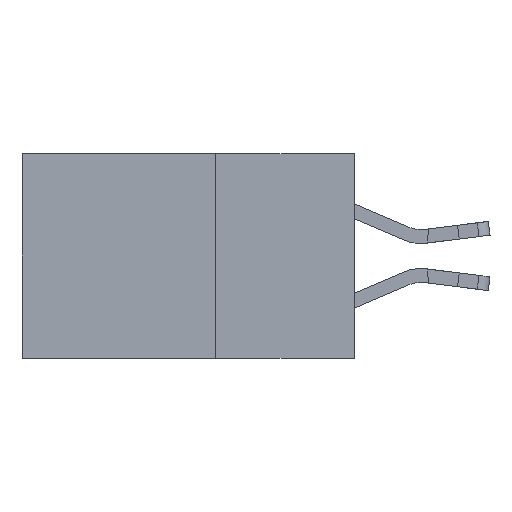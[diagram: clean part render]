
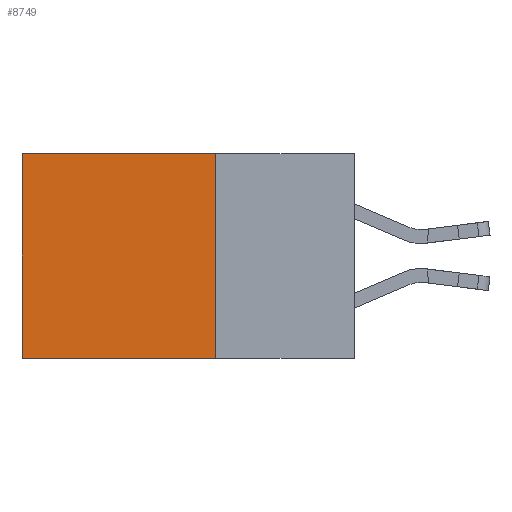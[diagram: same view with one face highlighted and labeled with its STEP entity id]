
A CAD part, left-side view. The second image highlights one B-rep face of the part: STEP entity #8749.
In plain terms, the highlighted planar face has unit normal (-1, 0, 0).
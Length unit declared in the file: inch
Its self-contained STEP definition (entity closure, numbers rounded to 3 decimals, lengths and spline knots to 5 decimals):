
#829 = EDGE_CURVE ( 'NONE', #6192, #14284, #8144, .T. ) ;
#2769 = CARTESIAN_POINT ( 'NONE',  ( 0.298, 0.6, -0.37 ) ) ;
#3401 = CARTESIAN_POINT ( 'NONE',  ( 0.298, 0.25, 0. ) ) ;
#4097 = LINE ( 'NONE', #3401, #11950 ) ;
#4464 = CARTESIAN_POINT ( 'NONE',  ( 0.298, 0.6, 0. ) ) ;
#4485 = LINE ( 'NONE', #6774, #6534 ) ;
#4515 = EDGE_CURVE ( 'NONE', #8010, #6192, #4485, .T. ) ;
#5329 = DIRECTION ( 'NONE',  ( 0., 1., 0. ) ) ;
#5430 = CARTESIAN_POINT ( 'NONE',  ( 0.298, 0.25, 0. ) ) ;
#6192 = VERTEX_POINT ( 'NONE', #6195 ) ;
#6195 = CARTESIAN_POINT ( 'NONE',  ( 0.298, 0.25, -0.37 ) ) ;
#6402 = CARTESIAN_POINT ( 'NONE',  ( 0.298, 0.6, 0. ) ) ;
#6466 = EDGE_CURVE ( 'NONE', #9532, #14284, #6539, .T. ) ;
#6534 = VECTOR ( 'NONE', #7986, 39.37008 ) ;
#6539 = LINE ( 'NONE', #4464, #15147 ) ;
#6612 = DIRECTION ( 'NONE',  ( 1., 0., 0. ) ) ;
#6774 = CARTESIAN_POINT ( 'NONE',  ( 0.298, 0.25, 0. ) ) ;
#6799 = EDGE_LOOP ( 'NONE', ( #9263, #11141, #10669, #11437 ) ) ;
#7322 = CARTESIAN_POINT ( 'NONE',  ( 0.298, 0.25, 0. ) ) ;
#7986 = DIRECTION ( 'NONE',  ( 0., 0., -1. ) ) ;
#8010 = VERTEX_POINT ( 'NONE', #7322 ) ;
#8144 = LINE ( 'NONE', #13534, #13372 ) ;
#8749 = ADVANCED_FACE ( 'NONE', ( #13050 ), #11327, .F. ) ;
#9263 = ORIENTED_EDGE ( 'NONE', *, *, #6466, .T. ) ;
#9532 = VERTEX_POINT ( 'NONE', #6402 ) ;
#10433 = DIRECTION ( 'NONE',  ( 0., 1., 0. ) ) ;
#10669 = ORIENTED_EDGE ( 'NONE', *, *, #4515, .F. ) ;
#11141 = ORIENTED_EDGE ( 'NONE', *, *, #829, .F. ) ;
#11327 = PLANE ( 'NONE',  #12902 ) ;
#11437 = ORIENTED_EDGE ( 'NONE', *, *, #14753, .T. ) ;
#11950 = VECTOR ( 'NONE', #10433, 39.37008 ) ;
#12640 = DIRECTION ( 'NONE',  ( 0., 0., -1. ) ) ;
#12902 = AXIS2_PLACEMENT_3D ( 'NONE', #5430, #6612, #12640 ) ;
#13050 = FACE_OUTER_BOUND ( 'NONE', #6799, .T. ) ;
#13372 = VECTOR ( 'NONE', #5329, 39.37008 ) ;
#13534 = CARTESIAN_POINT ( 'NONE',  ( 0.298, 0.25, -0.37 ) ) ;
#14284 = VERTEX_POINT ( 'NONE', #2769 ) ;
#14753 = EDGE_CURVE ( 'NONE', #8010, #9532, #4097, .T. ) ;
#15147 = VECTOR ( 'NONE', #15160, 39.37008 ) ;
#15160 = DIRECTION ( 'NONE',  ( 0., 0., -1. ) ) ;
